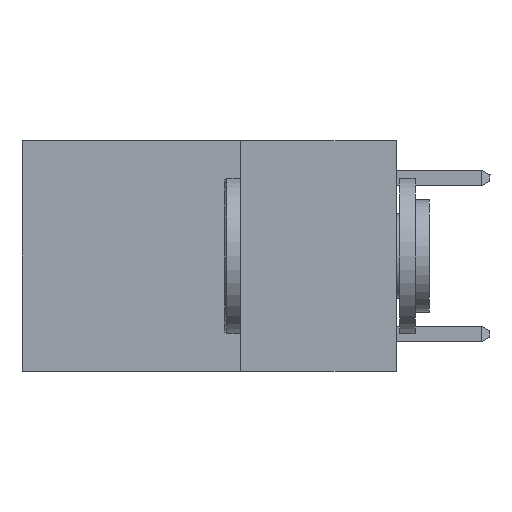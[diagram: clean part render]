
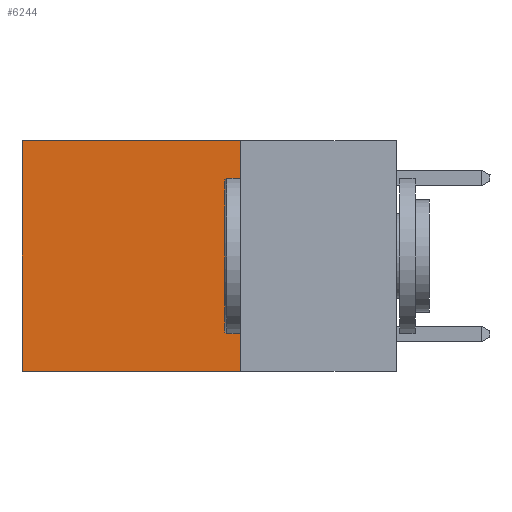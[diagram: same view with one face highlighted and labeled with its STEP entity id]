
A CAD part, left-side view. The second image highlights one B-rep face of the part: STEP entity #6244.
In plain terms, the highlighted planar face has unit normal (-1, 0, 0).
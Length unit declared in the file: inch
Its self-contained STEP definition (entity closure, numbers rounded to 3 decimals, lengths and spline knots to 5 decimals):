
#330 = VECTOR ( 'NONE', #12645, 39.37008 ) ;
#417 = ORIENTED_EDGE ( 'NONE', *, *, #10341, .T. ) ;
#1096 = DIRECTION ( 'NONE',  ( 0., 0., -1. ) ) ;
#1388 = VERTEX_POINT ( 'NONE', #12494 ) ;
#2769 = EDGE_CURVE ( 'NONE', #1388, #2861, #16206, .T. ) ;
#2861 = VERTEX_POINT ( 'NONE', #18148 ) ;
#4103 = VECTOR ( 'NONE', #11199, 39.37008 ) ;
#4570 = EDGE_CURVE ( 'NONE', #12712, #12130, #20810, .T. ) ;
#4678 = EDGE_LOOP ( 'NONE', ( #417, #9730, #9780, #11293 ) ) ;
#4866 = EDGE_CURVE ( 'NONE', #1388, #12712, #12007, .T. ) ;
#6098 = CARTESIAN_POINT ( 'NONE',  ( 0.2625, 0.25, -0.37 ) ) ;
#6215 = PLANE ( 'NONE',  #14149 ) ;
#6244 = ADVANCED_FACE ( 'NONE', ( #15731 ), #6215, .F. ) ;
#7712 = CARTESIAN_POINT ( 'NONE',  ( 0.2625, 0.25, 0. ) ) ;
#8760 = DIRECTION ( 'NONE',  ( 0., 0., -1. ) ) ;
#9730 = ORIENTED_EDGE ( 'NONE', *, *, #4570, .F. ) ;
#9780 = ORIENTED_EDGE ( 'NONE', *, *, #4866, .F. ) ;
#10341 = EDGE_CURVE ( 'NONE', #2861, #12130, #19487, .T. ) ;
#11199 = DIRECTION ( 'NONE',  ( 0., 1., 0. ) ) ;
#11293 = ORIENTED_EDGE ( 'NONE', *, *, #2769, .T. ) ;
#12007 = LINE ( 'NONE', #13888, #13099 ) ;
#12130 = VERTEX_POINT ( 'NONE', #20663 ) ;
#12494 = CARTESIAN_POINT ( 'NONE',  ( 0.2625, 0.25, 0. ) ) ;
#12645 = DIRECTION ( 'NONE',  ( 0., 1., 0. ) ) ;
#12712 = VERTEX_POINT ( 'NONE', #18030 ) ;
#12961 = DIRECTION ( 'NONE',  ( 0., 0., -1. ) ) ;
#13099 = VECTOR ( 'NONE', #8760, 39.37008 ) ;
#13888 = CARTESIAN_POINT ( 'NONE',  ( 0.2625, 0.25, 0. ) ) ;
#14149 = AXIS2_PLACEMENT_3D ( 'NONE', #7712, #18742, #1096 ) ;
#15217 = VECTOR ( 'NONE', #12961, 39.37008 ) ;
#15731 = FACE_OUTER_BOUND ( 'NONE', #4678, .T. ) ;
#16206 = LINE ( 'NONE', #19337, #4103 ) ;
#18030 = CARTESIAN_POINT ( 'NONE',  ( 0.2625, 0.25, -0.37 ) ) ;
#18148 = CARTESIAN_POINT ( 'NONE',  ( 0.2625, 0.6, 0. ) ) ;
#18742 = DIRECTION ( 'NONE',  ( 1., 0., 0. ) ) ;
#19337 = CARTESIAN_POINT ( 'NONE',  ( 0.2625, 0.25, 0. ) ) ;
#19487 = LINE ( 'NONE', #21012, #15217 ) ;
#20663 = CARTESIAN_POINT ( 'NONE',  ( 0.2625, 0.6, -0.37 ) ) ;
#20810 = LINE ( 'NONE', #6098, #330 ) ;
#21012 = CARTESIAN_POINT ( 'NONE',  ( 0.2625, 0.6, 0. ) ) ;
